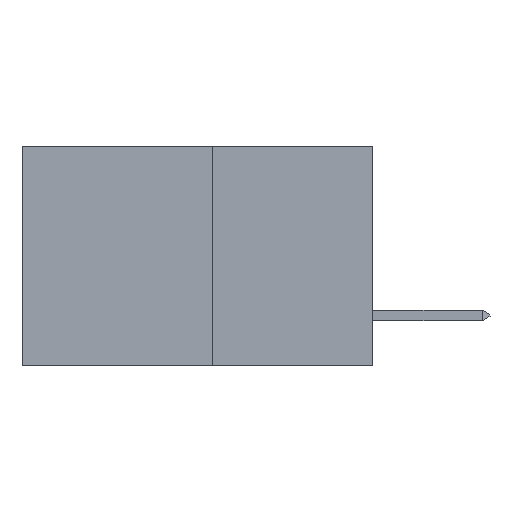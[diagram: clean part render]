
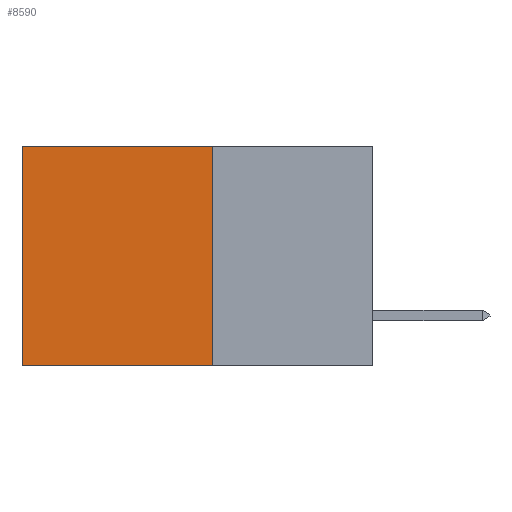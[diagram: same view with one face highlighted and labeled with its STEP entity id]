
A CAD part, left-side view. The second image highlights one B-rep face of the part: STEP entity #8590.
In plain terms, the highlighted planar face has unit normal (-1, 0, 0).
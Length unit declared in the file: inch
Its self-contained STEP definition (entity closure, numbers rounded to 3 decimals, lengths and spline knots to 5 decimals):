
#25 = LINE ( 'NONE', #8250, #8269 ) ;
#308 = LINE ( 'NONE', #2164, #8289 ) ;
#970 = DIRECTION ( 'NONE',  ( 0., 1., 0. ) ) ;
#1336 = CARTESIAN_POINT ( 'NONE',  ( 0.277, 0.59, 0. ) ) ;
#1443 = ORIENTED_EDGE ( 'NONE', *, *, #5290, .T. ) ;
#1753 = CARTESIAN_POINT ( 'NONE',  ( 0.277, 0.27, -0.37 ) ) ;
#2105 = ORIENTED_EDGE ( 'NONE', *, *, #4438, .T. ) ;
#2164 = CARTESIAN_POINT ( 'NONE',  ( 0.277, 0.27, 0. ) ) ;
#2490 = VECTOR ( 'NONE', #6941, 39.37008 ) ;
#2733 = ORIENTED_EDGE ( 'NONE', *, *, #5336, .F. ) ;
#2782 = DIRECTION ( 'NONE',  ( 1., 0., 0. ) ) ;
#3308 = FACE_OUTER_BOUND ( 'NONE', #4909, .T. ) ;
#3748 = EDGE_CURVE ( 'NONE', #5463, #7599, #6197, .T. ) ;
#3843 = CARTESIAN_POINT ( 'NONE',  ( 0.277, 0.27, -0.37 ) ) ;
#3932 = VERTEX_POINT ( 'NONE', #1336 ) ;
#4345 = LINE ( 'NONE', #7158, #8042 ) ;
#4438 = EDGE_CURVE ( 'NONE', #5195, #3932, #308, .T. ) ;
#4909 = EDGE_LOOP ( 'NONE', ( #1443, #9541, #2733, #2105 ) ) ;
#4949 = CARTESIAN_POINT ( 'NONE',  ( 0.277, 0.27, 0. ) ) ;
#5159 = CARTESIAN_POINT ( 'NONE',  ( 0.277, 0.27, -0.37 ) ) ;
#5195 = VERTEX_POINT ( 'NONE', #4949 ) ;
#5290 = EDGE_CURVE ( 'NONE', #3932, #7599, #25, .T. ) ;
#5336 = EDGE_CURVE ( 'NONE', #5195, #5463, #4345, .T. ) ;
#5463 = VERTEX_POINT ( 'NONE', #1753 ) ;
#5921 = AXIS2_PLACEMENT_3D ( 'NONE', #5159, #2782, #8295 ) ;
#6197 = LINE ( 'NONE', #3843, #2490 ) ;
#6941 = DIRECTION ( 'NONE',  ( 0., 1., 0. ) ) ;
#7051 = DIRECTION ( 'NONE',  ( 0., 0., -1. ) ) ;
#7158 = CARTESIAN_POINT ( 'NONE',  ( 0.277, 0.27, -0.37 ) ) ;
#7513 = PLANE ( 'NONE',  #5921 ) ;
#7599 = VERTEX_POINT ( 'NONE', #9275 ) ;
#8042 = VECTOR ( 'NONE', #7051, 39.37008 ) ;
#8055 = DIRECTION ( 'NONE',  ( 0., 0., -1. ) ) ;
#8250 = CARTESIAN_POINT ( 'NONE',  ( 0.277, 0.59, -0.37 ) ) ;
#8269 = VECTOR ( 'NONE', #8055, 39.37008 ) ;
#8289 = VECTOR ( 'NONE', #970, 39.37008 ) ;
#8295 = DIRECTION ( 'NONE',  ( 0., 0., -1. ) ) ;
#8590 = ADVANCED_FACE ( 'NONE', ( #3308 ), #7513, .F. ) ;
#9275 = CARTESIAN_POINT ( 'NONE',  ( 0.277, 0.59, -0.37 ) ) ;
#9541 = ORIENTED_EDGE ( 'NONE', *, *, #3748, .F. ) ;
